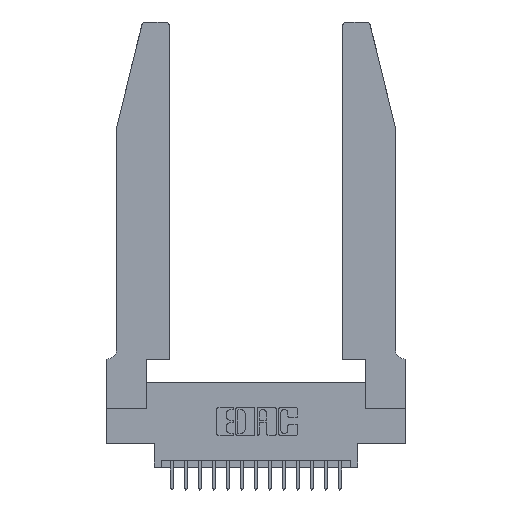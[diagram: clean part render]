
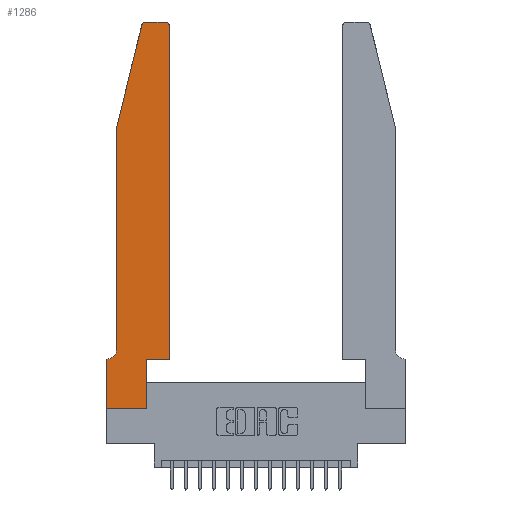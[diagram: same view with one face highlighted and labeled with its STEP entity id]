
A CAD part, top view. The second image highlights one B-rep face of the part: STEP entity #1286.
In plain terms, the highlighted planar face has unit normal (0, 0, 1).
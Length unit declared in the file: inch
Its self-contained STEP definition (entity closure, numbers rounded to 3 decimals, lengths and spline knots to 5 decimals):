
#140 = CIRCLE ( 'NONE', #12126, 0.03 ) ;
#312 = CARTESIAN_POINT ( 'NONE',  ( 0.0755, 0.35, 0.37 ) ) ;
#437 = ORIENTED_EDGE ( 'NONE', *, *, #4716, .T. ) ;
#472 = CARTESIAN_POINT ( 'NONE',  ( 0.2865, 0.35, 0.37 ) ) ;
#758 = DIRECTION ( 'NONE',  ( 1., 0., 0. ) ) ;
#901 = VERTEX_POINT ( 'NONE', #17008 ) ;
#1274 = AXIS2_PLACEMENT_3D ( 'NONE', #16930, #15586, #758 ) ;
#1286 = ADVANCED_FACE ( 'NONE', ( #12598 ), #2135, .T. ) ;
#1435 = VERTEX_POINT ( 'NONE', #11790 ) ;
#1776 = CARTESIAN_POINT ( 'NONE',  ( 0.0055, 0.35, 0.37 ) ) ;
#1797 = DIRECTION ( 'NONE',  ( 1., 0., 0. ) ) ;
#2135 = PLANE ( 'NONE',  #17390 ) ;
#2221 = CARTESIAN_POINT ( 'NONE',  ( 0., 0., 0.37 ) ) ;
#2571 = VERTEX_POINT ( 'NONE', #16402 ) ;
#2938 = CARTESIAN_POINT ( 'NONE',  ( 0.0755, 2., 0.37 ) ) ;
#3080 = VECTOR ( 'NONE', #3636, 39.37008 ) ;
#3148 = VERTEX_POINT ( 'NONE', #13109 ) ;
#3378 = VERTEX_POINT ( 'NONE', #2938 ) ;
#3468 = LINE ( 'NONE', #13891, #8313 ) ;
#3577 = LINE ( 'NONE', #16039, #8196 ) ;
#3636 = DIRECTION ( 'NONE',  ( 0., -1., 0. ) ) ;
#4307 = CARTESIAN_POINT ( 'NONE',  ( 0.0755, 0.42, 0.37 ) ) ;
#4377 = EDGE_LOOP ( 'NONE', ( #18849, #15055, #16411, #18425, #437, #9848, #7498, #10167, #8507, #16625, #18787, #6165 ) ) ;
#4710 = EDGE_CURVE ( 'NONE', #16663, #901, #15156, .T. ) ;
#4716 = EDGE_CURVE ( 'NONE', #17298, #18996, #6345, .T. ) ;
#5516 = CARTESIAN_POINT ( 'NONE',  ( 0., 0., 0.37 ) ) ;
#5777 = LINE ( 'NONE', #472, #11073 ) ;
#5808 = VECTOR ( 'NONE', #14104, 39.37008 ) ;
#6165 = ORIENTED_EDGE ( 'NONE', *, *, #13067, .T. ) ;
#6345 = CIRCLE ( 'NONE', #12324, 0.07 ) ;
#6867 = LINE ( 'NONE', #8155, #5808 ) ;
#7498 = ORIENTED_EDGE ( 'NONE', *, *, #14763, .T. ) ;
#7737 = VECTOR ( 'NONE', #17450, 39.37008 ) ;
#8010 = DIRECTION ( 'NONE',  ( -0.239, -0.971, 0. ) ) ;
#8081 = DIRECTION ( 'NONE',  ( 0., -1., 0. ) ) ;
#8125 = DIRECTION ( 'NONE',  ( 0., 1., 0. ) ) ;
#8155 = CARTESIAN_POINT ( 'NONE',  ( 0.4505, 0.35, 0.37 ) ) ;
#8196 = VECTOR ( 'NONE', #18990, 39.37008 ) ;
#8313 = VECTOR ( 'NONE', #8081, 39.37008 ) ;
#8507 = ORIENTED_EDGE ( 'NONE', *, *, #16471, .T. ) ;
#8774 = DIRECTION ( 'NONE',  ( 0., 0., -1. ) ) ;
#9378 = CARTESIAN_POINT ( 'NONE',  ( 0.25487, 2.72718, 0.37 ) ) ;
#9664 = DIRECTION ( 'NONE',  ( 0., 0., 1. ) ) ;
#9825 = VECTOR ( 'NONE', #8010, 39.37008 ) ;
#9848 = ORIENTED_EDGE ( 'NONE', *, *, #10275, .T. ) ;
#9862 = CARTESIAN_POINT ( 'NONE',  ( 0.4205, 2.75, 0.37 ) ) ;
#9961 = CARTESIAN_POINT ( 'NONE',  ( 0.4205, 2.72, 0.37 ) ) ;
#10024 = DIRECTION ( 'NONE',  ( 1., 0., 0. ) ) ;
#10167 = ORIENTED_EDGE ( 'NONE', *, *, #14077, .T. ) ;
#10275 = EDGE_CURVE ( 'NONE', #18996, #13362, #14947, .T. ) ;
#10361 = VERTEX_POINT ( 'NONE', #12845 ) ;
#10398 = DIRECTION ( 'NONE',  ( -1., 0., 0. ) ) ;
#10487 = EDGE_CURVE ( 'NONE', #2571, #10361, #6867, .T. ) ;
#10699 = CARTESIAN_POINT ( 'NONE',  ( 0., 0.35, 0.37 ) ) ;
#10703 = CIRCLE ( 'NONE', #1274, 0.03 ) ;
#11073 = VECTOR ( 'NONE', #8125, 39.37008 ) ;
#11144 = LINE ( 'NONE', #2221, #3080 ) ;
#11790 = CARTESIAN_POINT ( 'NONE',  ( 0.4505, 2.72, 0.37 ) ) ;
#11976 = DIRECTION ( 'NONE',  ( -1., 0., 0. ) ) ;
#12126 = AXIS2_PLACEMENT_3D ( 'NONE', #9961, #12922, #10024 ) ;
#12164 = CARTESIAN_POINT ( 'NONE',  ( 0.0755, 2., 0.37 ) ) ;
#12240 = EDGE_CURVE ( 'NONE', #15746, #3378, #13732, .T. ) ;
#12324 = AXIS2_PLACEMENT_3D ( 'NONE', #17877, #8774, #10398 ) ;
#12598 = FACE_OUTER_BOUND ( 'NONE', #4377, .T. ) ;
#12691 = VERTEX_POINT ( 'NONE', #5516 ) ;
#12845 = CARTESIAN_POINT ( 'NONE',  ( 0.4505, 0.35, 0.37 ) ) ;
#12863 = EDGE_CURVE ( 'NONE', #901, #15746, #10703, .T. ) ;
#12893 = DIRECTION ( 'NONE',  ( 1., 0., 0. ) ) ;
#12914 = CARTESIAN_POINT ( 'NONE',  ( 0.2605, 2.75, 0.37 ) ) ;
#12922 = DIRECTION ( 'NONE',  ( 0., 0., 1. ) ) ;
#13067 = EDGE_CURVE ( 'NONE', #1435, #16663, #140, .T. ) ;
#13109 = CARTESIAN_POINT ( 'NONE',  ( 0.2865, 0., 0.37 ) ) ;
#13130 = EDGE_CURVE ( 'NONE', #10361, #1435, #3577, .T. ) ;
#13362 = VERTEX_POINT ( 'NONE', #10699 ) ;
#13732 = LINE ( 'NONE', #12164, #9825 ) ;
#13891 = CARTESIAN_POINT ( 'NONE',  ( 0.0755, 2., 0.37 ) ) ;
#14077 = EDGE_CURVE ( 'NONE', #12691, #3148, #16487, .T. ) ;
#14104 = DIRECTION ( 'NONE',  ( 1., 0., 0. ) ) ;
#14763 = EDGE_CURVE ( 'NONE', #13362, #12691, #11144, .T. ) ;
#14947 = LINE ( 'NONE', #312, #16322 ) ;
#15055 = ORIENTED_EDGE ( 'NONE', *, *, #12863, .T. ) ;
#15156 = LINE ( 'NONE', #12914, #7737 ) ;
#15586 = DIRECTION ( 'NONE',  ( 0., 0., 1. ) ) ;
#15746 = VERTEX_POINT ( 'NONE', #9378 ) ;
#16008 = EDGE_CURVE ( 'NONE', #3378, #17298, #3468, .T. ) ;
#16039 = CARTESIAN_POINT ( 'NONE',  ( 0.4505, 0.35, 0.37 ) ) ;
#16322 = VECTOR ( 'NONE', #11976, 39.37008 ) ;
#16402 = CARTESIAN_POINT ( 'NONE',  ( 0.2865, 0.35, 0.37 ) ) ;
#16411 = ORIENTED_EDGE ( 'NONE', *, *, #12240, .T. ) ;
#16471 = EDGE_CURVE ( 'NONE', #3148, #2571, #5777, .T. ) ;
#16487 = LINE ( 'NONE', #16740, #18083 ) ;
#16625 = ORIENTED_EDGE ( 'NONE', *, *, #10487, .T. ) ;
#16663 = VERTEX_POINT ( 'NONE', #9862 ) ;
#16740 = CARTESIAN_POINT ( 'NONE',  ( 0., 0., 0.37 ) ) ;
#16930 = CARTESIAN_POINT ( 'NONE',  ( 0.284, 2.72, 0.37 ) ) ;
#17008 = CARTESIAN_POINT ( 'NONE',  ( 0.284, 2.75, 0.37 ) ) ;
#17298 = VERTEX_POINT ( 'NONE', #4307 ) ;
#17390 = AXIS2_PLACEMENT_3D ( 'NONE', #18442, #9664, #12893 ) ;
#17450 = DIRECTION ( 'NONE',  ( -1., 0., 0. ) ) ;
#17877 = CARTESIAN_POINT ( 'NONE',  ( 0.0055, 0.42, 0.37 ) ) ;
#18083 = VECTOR ( 'NONE', #1797, 39.37008 ) ;
#18425 = ORIENTED_EDGE ( 'NONE', *, *, #16008, .T. ) ;
#18442 = CARTESIAN_POINT ( 'NONE',  ( 0., 0.35, 0.37 ) ) ;
#18787 = ORIENTED_EDGE ( 'NONE', *, *, #13130, .T. ) ;
#18849 = ORIENTED_EDGE ( 'NONE', *, *, #4710, .T. ) ;
#18990 = DIRECTION ( 'NONE',  ( 0., 1., 0. ) ) ;
#18996 = VERTEX_POINT ( 'NONE', #1776 ) ;
